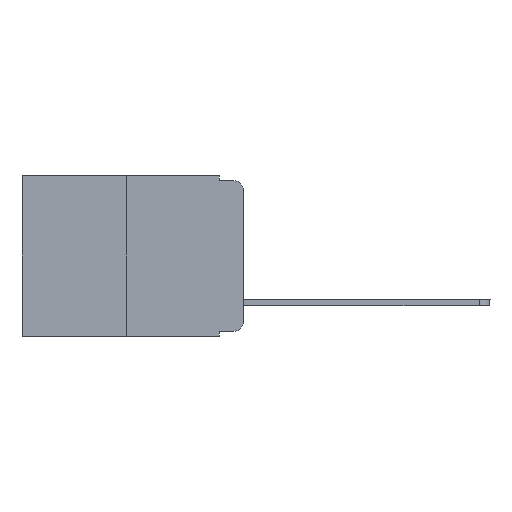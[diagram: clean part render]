
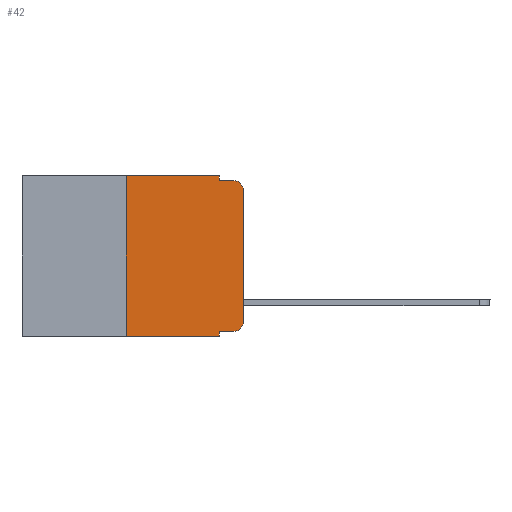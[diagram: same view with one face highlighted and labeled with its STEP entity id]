
A CAD part, left-side view. The second image highlights one B-rep face of the part: STEP entity #42.
In plain terms, the highlighted planar face has unit normal (-1, 0, 0).
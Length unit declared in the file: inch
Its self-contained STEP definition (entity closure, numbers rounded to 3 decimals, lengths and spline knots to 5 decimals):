
#42 = ADVANCED_FACE ( 'NONE', ( #19457 ), #2876, .F. ) ;
#182 = EDGE_CURVE ( 'NONE', #14409, #19900, #18114, .T. ) ;
#286 = VECTOR ( 'NONE', #17343, 39.37008 ) ;
#819 = LINE ( 'NONE', #7793, #17001 ) ;
#1021 = EDGE_CURVE ( 'NONE', #2263, #18544, #7693, .T. ) ;
#1449 = VECTOR ( 'NONE', #10766, 39.37008 ) ;
#1592 = VECTOR ( 'NONE', #7931, 39.37008 ) ;
#2043 = CARTESIAN_POINT ( 'NONE',  ( 0., 0., -0.313 ) ) ;
#2244 = EDGE_CURVE ( 'NONE', #8615, #18376, #10552, .T. ) ;
#2263 = VERTEX_POINT ( 'NONE', #2043 ) ;
#2876 = PLANE ( 'NONE',  #18591 ) ;
#3763 = EDGE_LOOP ( 'NONE', ( #7382, #17572, #7476, #23762, #5778, #7962, #19134, #23539, #12407, #8585 ) ) ;
#4403 = DIRECTION ( 'NONE',  ( 0., -1., 0. ) ) ;
#4429 = CARTESIAN_POINT ( 'NONE',  ( 0., 0., 0. ) ) ;
#4558 = EDGE_CURVE ( 'NONE', #8615, #19395, #15498, .T. ) ;
#4689 = VECTOR ( 'NONE', #16052, 39.37008 ) ;
#5293 = EDGE_CURVE ( 'NONE', #18544, #20497, #9614, .T. ) ;
#5363 = DIRECTION ( 'NONE',  ( 0., 0., -1. ) ) ;
#5397 = CARTESIAN_POINT ( 'NONE',  ( 0., 0.25, 0. ) ) ;
#5778 = ORIENTED_EDGE ( 'NONE', *, *, #8673, .F. ) ;
#6268 = DIRECTION ( 'NONE',  ( 0., -1., 0. ) ) ;
#6567 = CIRCLE ( 'NONE', #20125, 0.02 ) ;
#6591 = DIRECTION ( 'NONE',  ( 1., 0., 0. ) ) ;
#6711 = CARTESIAN_POINT ( 'NONE',  ( 0., 0.051, -0.333 ) ) ;
#6931 = VERTEX_POINT ( 'NONE', #13328 ) ;
#7382 = ORIENTED_EDGE ( 'NONE', *, *, #1021, .T. ) ;
#7476 = ORIENTED_EDGE ( 'NONE', *, *, #15729, .F. ) ;
#7523 = CARTESIAN_POINT ( 'NONE',  ( 0., 0.02, -0.03 ) ) ;
#7693 = LINE ( 'NONE', #4429, #1592 ) ;
#7793 = CARTESIAN_POINT ( 'NONE',  ( 0., 0.051, -0.333 ) ) ;
#7931 = DIRECTION ( 'NONE',  ( 0., 0., 1. ) ) ;
#7962 = ORIENTED_EDGE ( 'NONE', *, *, #2244, .F. ) ;
#8085 = DIRECTION ( 'NONE',  ( 0., 0., -1. ) ) ;
#8585 = ORIENTED_EDGE ( 'NONE', *, *, #12599, .T. ) ;
#8615 = VERTEX_POINT ( 'NONE', #13342 ) ;
#8673 = EDGE_CURVE ( 'NONE', #18376, #14409, #19396, .T. ) ;
#8744 = CARTESIAN_POINT ( 'NONE',  ( 0., 0.051, 0. ) ) ;
#9614 = CIRCLE ( 'NONE', #16191, 0.02 ) ;
#10552 = LINE ( 'NONE', #16368, #1449 ) ;
#10766 = DIRECTION ( 'NONE',  ( 0., 0., 1. ) ) ;
#11534 = CARTESIAN_POINT ( 'NONE',  ( 0., 0.051, 0. ) ) ;
#11557 = EDGE_CURVE ( 'NONE', #12946, #6931, #819, .T. ) ;
#12086 = CARTESIAN_POINT ( 'NONE',  ( 0., 0.051, -0.01 ) ) ;
#12407 = ORIENTED_EDGE ( 'NONE', *, *, #11557, .T. ) ;
#12503 = CARTESIAN_POINT ( 'NONE',  ( 0., 0.02, -0.01 ) ) ;
#12599 = EDGE_CURVE ( 'NONE', #6931, #2263, #6567, .T. ) ;
#12946 = VERTEX_POINT ( 'NONE', #6711 ) ;
#13095 = CARTESIAN_POINT ( 'NONE',  ( 0., 0.051, -0.343 ) ) ;
#13328 = CARTESIAN_POINT ( 'NONE',  ( 0., 0.02, -0.333 ) ) ;
#13342 = CARTESIAN_POINT ( 'NONE',  ( 0., 0.25, -0.343 ) ) ;
#13826 = CARTESIAN_POINT ( 'NONE',  ( 0., 0.473, 0. ) ) ;
#13907 = CARTESIAN_POINT ( 'NONE',  ( 0., 0.473, -0.343 ) ) ;
#14409 = VERTEX_POINT ( 'NONE', #11534 ) ;
#14824 = EDGE_CURVE ( 'NONE', #12946, #19395, #21847, .T. ) ;
#14937 = DIRECTION ( 'NONE',  ( -1., 0., 0. ) ) ;
#15498 = LINE ( 'NONE', #13907, #19236 ) ;
#15729 = EDGE_CURVE ( 'NONE', #19900, #20497, #23250, .T. ) ;
#16052 = DIRECTION ( 'NONE',  ( 0., 0., -1. ) ) ;
#16191 = AXIS2_PLACEMENT_3D ( 'NONE', #7523, #14937, #5363 ) ;
#16368 = CARTESIAN_POINT ( 'NONE',  ( 0., 0.25, 0. ) ) ;
#17001 = VECTOR ( 'NONE', #4403, 39.37008 ) ;
#17343 = DIRECTION ( 'NONE',  ( 0., -1., 0. ) ) ;
#17572 = ORIENTED_EDGE ( 'NONE', *, *, #5293, .T. ) ;
#18114 = LINE ( 'NONE', #18244, #21671 ) ;
#18244 = CARTESIAN_POINT ( 'NONE',  ( 0., 0.051, 0. ) ) ;
#18348 = DIRECTION ( 'NONE',  ( 0., 0., -1. ) ) ;
#18376 = VERTEX_POINT ( 'NONE', #5397 ) ;
#18544 = VERTEX_POINT ( 'NONE', #19456 ) ;
#18591 = AXIS2_PLACEMENT_3D ( 'NONE', #19211, #6591, #19573 ) ;
#19134 = ORIENTED_EDGE ( 'NONE', *, *, #4558, .T. ) ;
#19211 = CARTESIAN_POINT ( 'NONE',  ( 0., 0.473, 0. ) ) ;
#19236 = VECTOR ( 'NONE', #6268, 39.37008 ) ;
#19395 = VERTEX_POINT ( 'NONE', #13095 ) ;
#19396 = LINE ( 'NONE', #13826, #286 ) ;
#19456 = CARTESIAN_POINT ( 'NONE',  ( 0., 0., -0.03 ) ) ;
#19457 = FACE_OUTER_BOUND ( 'NONE', #3763, .T. ) ;
#19573 = DIRECTION ( 'NONE',  ( 0., 0., -1. ) ) ;
#19731 = CARTESIAN_POINT ( 'NONE',  ( 0., 0.02, -0.313 ) ) ;
#19900 = VERTEX_POINT ( 'NONE', #12086 ) ;
#20125 = AXIS2_PLACEMENT_3D ( 'NONE', #19731, #21069, #8085 ) ;
#20497 = VERTEX_POINT ( 'NONE', #12503 ) ;
#21069 = DIRECTION ( 'NONE',  ( -1., 0., 0. ) ) ;
#21671 = VECTOR ( 'NONE', #18348, 39.37008 ) ;
#21847 = LINE ( 'NONE', #8744, #4689 ) ;
#22124 = VECTOR ( 'NONE', #23002, 39.37008 ) ;
#23002 = DIRECTION ( 'NONE',  ( 0., -1., 0. ) ) ;
#23119 = CARTESIAN_POINT ( 'NONE',  ( 0., 0.051, -0.01 ) ) ;
#23250 = LINE ( 'NONE', #23119, #22124 ) ;
#23539 = ORIENTED_EDGE ( 'NONE', *, *, #14824, .F. ) ;
#23762 = ORIENTED_EDGE ( 'NONE', *, *, #182, .F. ) ;
